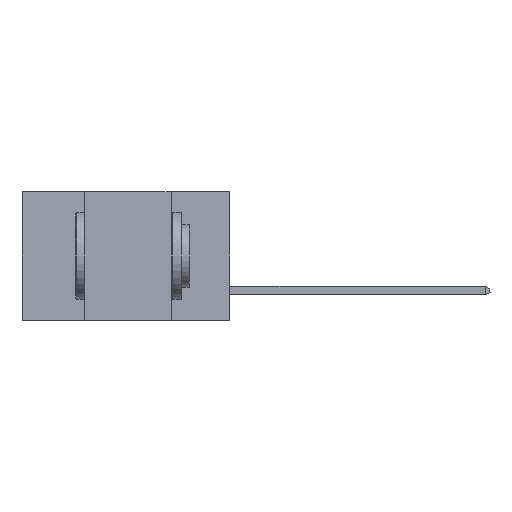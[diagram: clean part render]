
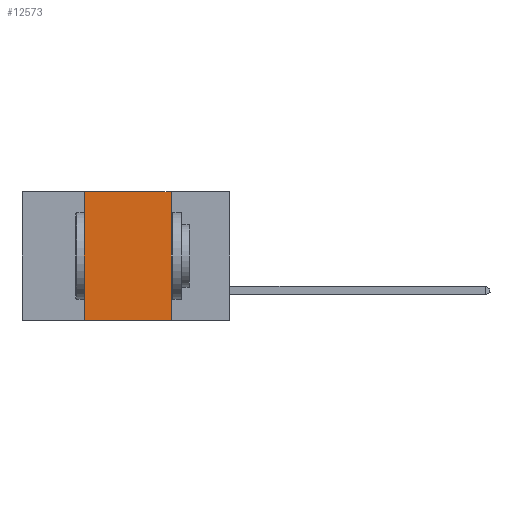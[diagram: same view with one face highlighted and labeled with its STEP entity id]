
A CAD part, left-side view. The second image highlights one B-rep face of the part: STEP entity #12573.
In plain terms, the highlighted planar face has unit normal (-1, 0, 0).
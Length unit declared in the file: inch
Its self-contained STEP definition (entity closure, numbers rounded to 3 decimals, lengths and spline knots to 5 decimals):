
#1444 = EDGE_CURVE ( 'NONE', #18690, #23239, #13462, .T. ) ;
#1537 = EDGE_CURVE ( 'NONE', #7420, #15047, #10977, .T. ) ;
#1827 = LINE ( 'NONE', #21380, #9272 ) ;
#3969 = DIRECTION ( 'NONE',  ( 0., 0., -1. ) ) ;
#4611 = ORIENTED_EDGE ( 'NONE', *, *, #1537, .F. ) ;
#4638 = EDGE_CURVE ( 'NONE', #7420, #23239, #11571, .T. ) ;
#4657 = DIRECTION ( 'NONE',  ( 0., -1., 0. ) ) ;
#4899 = CARTESIAN_POINT ( 'NONE',  ( 0., 0.42, 0. ) ) ;
#5198 = CARTESIAN_POINT ( 'NONE',  ( 0., 0.6, 0. ) ) ;
#7420 = VERTEX_POINT ( 'NONE', #12617 ) ;
#8741 = FACE_OUTER_BOUND ( 'NONE', #27039, .T. ) ;
#8944 = CARTESIAN_POINT ( 'NONE',  ( 0., 0.17, 0. ) ) ;
#9204 = ORIENTED_EDGE ( 'NONE', *, *, #4638, .T. ) ;
#9272 = VECTOR ( 'NONE', #14620, 39.37008 ) ;
#10977 = LINE ( 'NONE', #4899, #19841 ) ;
#11571 = LINE ( 'NONE', #21405, #22200 ) ;
#12142 = DIRECTION ( 'NONE',  ( 0., 0., 1. ) ) ;
#12573 = ADVANCED_FACE ( 'NONE', ( #8741 ), #23470, .F. ) ;
#12617 = CARTESIAN_POINT ( 'NONE',  ( 0., 0.42, -0.37 ) ) ;
#13462 = LINE ( 'NONE', #22336, #16312 ) ;
#14576 = ORIENTED_EDGE ( 'NONE', *, *, #1444, .F. ) ;
#14620 = DIRECTION ( 'NONE',  ( 0., -1., 0. ) ) ;
#14984 = EDGE_CURVE ( 'NONE', #15047, #18690, #1827, .T. ) ;
#15047 = VERTEX_POINT ( 'NONE', #28322 ) ;
#15626 = CARTESIAN_POINT ( 'NONE',  ( 0., 0.17, -0.37 ) ) ;
#16312 = VECTOR ( 'NONE', #3969, 39.37008 ) ;
#18690 = VERTEX_POINT ( 'NONE', #8944 ) ;
#19057 = DIRECTION ( 'NONE',  ( 1., 0., 0. ) ) ;
#19219 = ORIENTED_EDGE ( 'NONE', *, *, #14984, .F. ) ;
#19841 = VECTOR ( 'NONE', #12142, 39.37008 ) ;
#21380 = CARTESIAN_POINT ( 'NONE',  ( 0., 0.6, 0. ) ) ;
#21405 = CARTESIAN_POINT ( 'NONE',  ( 0., 0.6, -0.37 ) ) ;
#22200 = VECTOR ( 'NONE', #4657, 39.37008 ) ;
#22336 = CARTESIAN_POINT ( 'NONE',  ( 0., 0.17, 0. ) ) ;
#23239 = VERTEX_POINT ( 'NONE', #15626 ) ;
#23470 = PLANE ( 'NONE',  #27576 ) ;
#27039 = EDGE_LOOP ( 'NONE', ( #14576, #19219, #4611, #9204 ) ) ;
#27576 = AXIS2_PLACEMENT_3D ( 'NONE', #5198, #19057, #27980 ) ;
#27980 = DIRECTION ( 'NONE',  ( 0., 0., -1. ) ) ;
#28322 = CARTESIAN_POINT ( 'NONE',  ( 0., 0.42, 0. ) ) ;
